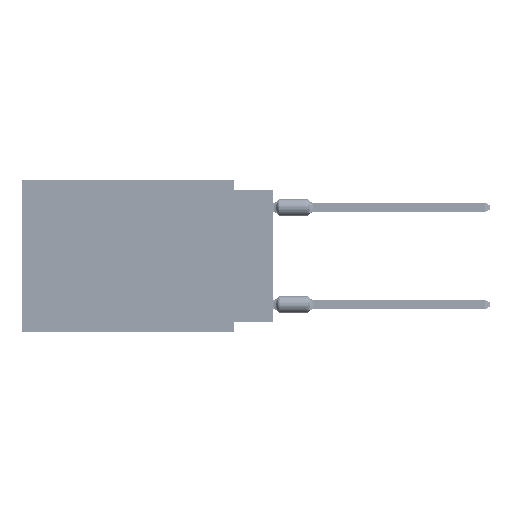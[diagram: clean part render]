
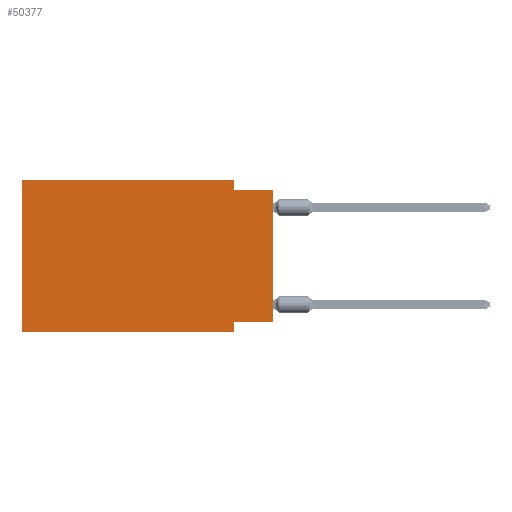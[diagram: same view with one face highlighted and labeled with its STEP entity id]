
A CAD part, left-side view. The second image highlights one B-rep face of the part: STEP entity #50377.
In plain terms, the highlighted planar face has unit normal (-1, 0, 0).
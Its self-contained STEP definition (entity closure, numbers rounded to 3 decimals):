
#499 = CARTESIAN_POINT ( 'NONE',  ( 0., 2.54, -9.906 ) ) ;
#4057 = ORIENTED_EDGE ( 'NONE', *, *, #73622, .F. ) ;
#4147 = CARTESIAN_POINT ( 'NONE',  ( 0., 0., -0.635 ) ) ;
#4559 = DIRECTION ( 'NONE',  ( 0., 0., -1. ) ) ;
#4812 = CARTESIAN_POINT ( 'NONE',  ( 0., 0., -0.635 ) ) ;
#5790 = DIRECTION ( 'NONE',  ( 1., 0., 0. ) ) ;
#5792 = LINE ( 'NONE', #72220, #81501 ) ;
#9094 = CARTESIAN_POINT ( 'NONE',  ( 0., 16.383, 0. ) ) ;
#9461 = VECTOR ( 'NONE', #18700, 1000. ) ;
#10664 = CARTESIAN_POINT ( 'NONE',  ( 0., 2.54, 0. ) ) ;
#10706 = VERTEX_POINT ( 'NONE', #4147 ) ;
#12043 = DIRECTION ( 'NONE',  ( 0., 0., 1. ) ) ;
#12065 = CARTESIAN_POINT ( 'NONE',  ( 0., 2.54, -9.271 ) ) ;
#12638 = VECTOR ( 'NONE', #4559, 1000. ) ;
#13176 = DIRECTION ( 'NONE',  ( 0., 0., 1. ) ) ;
#13772 = ORIENTED_EDGE ( 'NONE', *, *, #82203, .F. ) ;
#15192 = ORIENTED_EDGE ( 'NONE', *, *, #78215, .F. ) ;
#16518 = DIRECTION ( 'NONE',  ( 0., 0., -1. ) ) ;
#18235 = AXIS2_PLACEMENT_3D ( 'NONE', #59190, #5790, #78310 ) ;
#18259 = LINE ( 'NONE', #36135, #20382 ) ;
#18700 = DIRECTION ( 'NONE',  ( 0., -1., 0. ) ) ;
#19812 = VECTOR ( 'NONE', #12043, 1000. ) ;
#20382 = VECTOR ( 'NONE', #26947, 1000. ) ;
#21189 = VERTEX_POINT ( 'NONE', #26239 ) ;
#22642 = EDGE_CURVE ( 'NONE', #21189, #46850, #41685, .T. ) ;
#22913 = VERTEX_POINT ( 'NONE', #12065 ) ;
#23025 = CARTESIAN_POINT ( 'NONE',  ( 0., 2.54, -9.906 ) ) ;
#26239 = CARTESIAN_POINT ( 'NONE',  ( 0., 16.383, 0. ) ) ;
#26947 = DIRECTION ( 'NONE',  ( 0., 1., 0. ) ) ;
#27733 = ORIENTED_EDGE ( 'NONE', *, *, #71324, .F. ) ;
#28612 = CARTESIAN_POINT ( 'NONE',  ( 0., 2.54, -0.635 ) ) ;
#29871 = EDGE_CURVE ( 'NONE', #41035, #10706, #65180, .T. ) ;
#34939 = VECTOR ( 'NONE', #57228, 1000. ) ;
#36135 = CARTESIAN_POINT ( 'NONE',  ( 0., 0., -9.271 ) ) ;
#41035 = VERTEX_POINT ( 'NONE', #28612 ) ;
#41685 = LINE ( 'NONE', #9094, #70827 ) ;
#41739 = CARTESIAN_POINT ( 'NONE',  ( 0., 2.54, 0. ) ) ;
#42549 = CARTESIAN_POINT ( 'NONE',  ( 0., 16.383, -9.906 ) ) ;
#45933 = VERTEX_POINT ( 'NONE', #46668 ) ;
#46668 = CARTESIAN_POINT ( 'NONE',  ( 0., 16.383, -9.906 ) ) ;
#46850 = VERTEX_POINT ( 'NONE', #41739 ) ;
#49485 = LINE ( 'NONE', #42549, #34939 ) ;
#50377 = ADVANCED_FACE ( 'NONE', ( #65285 ), #70919, .F. ) ;
#50717 = CARTESIAN_POINT ( 'NONE',  ( 0., 16.383, 0. ) ) ;
#57228 = DIRECTION ( 'NONE',  ( 0., -1., 0. ) ) ;
#59190 = CARTESIAN_POINT ( 'NONE',  ( 0., 16.383, 0. ) ) ;
#62140 = EDGE_LOOP ( 'NONE', ( #67975, #74002, #27733, #82819, #4057, #82307, #13772, #15192 ) ) ;
#65180 = LINE ( 'NONE', #4812, #9461 ) ;
#65285 = FACE_OUTER_BOUND ( 'NONE', #62140, .T. ) ;
#67975 = ORIENTED_EDGE ( 'NONE', *, *, #79122, .T. ) ;
#68475 = CARTESIAN_POINT ( 'NONE',  ( 0., 0., -9.271 ) ) ;
#70827 = VECTOR ( 'NONE', #83310, 1000. ) ;
#70919 = PLANE ( 'NONE',  #18235 ) ;
#71324 = EDGE_CURVE ( 'NONE', #46850, #41035, #77518, .T. ) ;
#72058 = EDGE_CURVE ( 'NONE', #45933, #83249, #49485, .T. ) ;
#72220 = CARTESIAN_POINT ( 'NONE',  ( 0., 0., 0. ) ) ;
#73622 = EDGE_CURVE ( 'NONE', #45933, #21189, #84559, .T. ) ;
#74002 = ORIENTED_EDGE ( 'NONE', *, *, #29871, .F. ) ;
#77518 = LINE ( 'NONE', #10664, #12638 ) ;
#78215 = EDGE_CURVE ( 'NONE', #78779, #22913, #18259, .T. ) ;
#78310 = DIRECTION ( 'NONE',  ( 0., 0., -1. ) ) ;
#78779 = VERTEX_POINT ( 'NONE', #68475 ) ;
#79122 = EDGE_CURVE ( 'NONE', #78779, #10706, #5792, .T. ) ;
#81501 = VECTOR ( 'NONE', #13176, 1000. ) ;
#82203 = EDGE_CURVE ( 'NONE', #22913, #83249, #84218, .T. ) ;
#82307 = ORIENTED_EDGE ( 'NONE', *, *, #72058, .T. ) ;
#82819 = ORIENTED_EDGE ( 'NONE', *, *, #22642, .F. ) ;
#83249 = VERTEX_POINT ( 'NONE', #499 ) ;
#83310 = DIRECTION ( 'NONE',  ( 0., -1., 0. ) ) ;
#84218 = LINE ( 'NONE', #23025, #84409 ) ;
#84409 = VECTOR ( 'NONE', #16518, 1000. ) ;
#84559 = LINE ( 'NONE', #50717, #19812 ) ;
